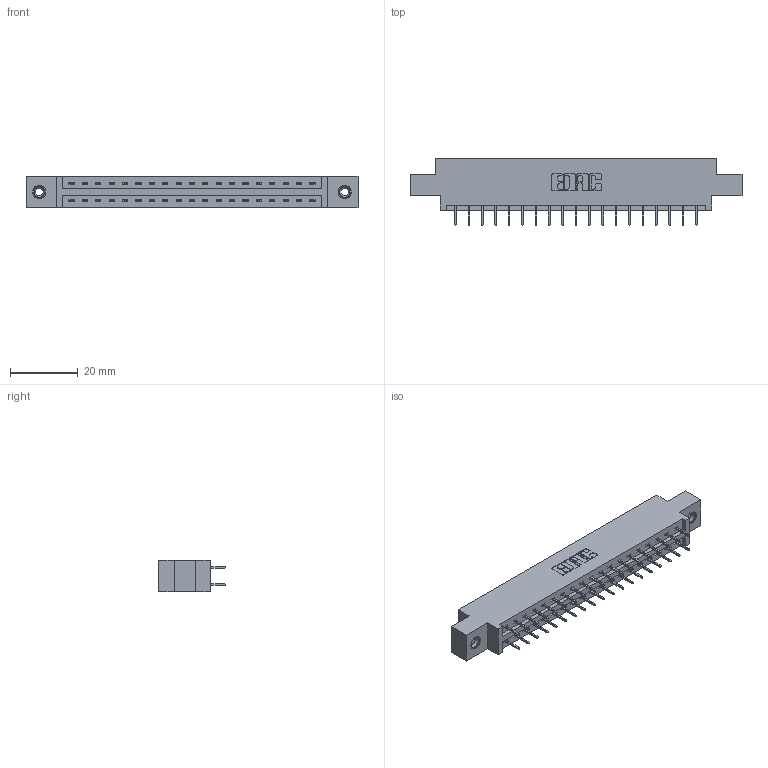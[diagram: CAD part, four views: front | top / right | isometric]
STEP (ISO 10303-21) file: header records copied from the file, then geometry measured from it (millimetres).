
FILE_DESCRIPTION (( 'STEP AP203' ), '1' );
FILE_NAME ('387-038-524-808.STEP', '2018-09-19T04:47:51', ( '' ), ( '' ), 'SwSTEP 2.0', 'SolidWorks 2016', '' );
FILE_SCHEMA (( 'CONFIG_CONTROL_DESIGN' ));
Length unit declared in the file: inch
Products named in the file (4): 387-038-524-808; 337 Part_0.170 Offset - 0.156 Dia-TI; 345-292-001_345-293-124; 345-250-001_345-250-003-102
Assembly tree (41 placements, depth 2):
  387-038-524-808
    337 Part_0.170 Offset - 0.156 Dia-TI
    345-292-001_345-293-124  x38
    345-250-001_345-250-003-102  x2
Bounding box: 98.3 x 19.69 x 9.4 mm (x, y, z)
Volume: 9871.7 mm3; surface area: 10890.3 mm2
Topology: 41 solids, 41 shells, 2382 faces, 6729 edges, 4326 vertices
Faces by surface type: plane 1778, cylinder 588, cone 12, torus 4
Entity records: 19098 total; most frequent: CARTESIAN_POINT 3217, ORIENTED_EDGE 3146, DIRECTION 2811, EDGE_CURVE 1573, VECTOR 1429, LINE 1429, VERTEX_POINT 1040, AXIS2_PLACEMENT_3D 691
